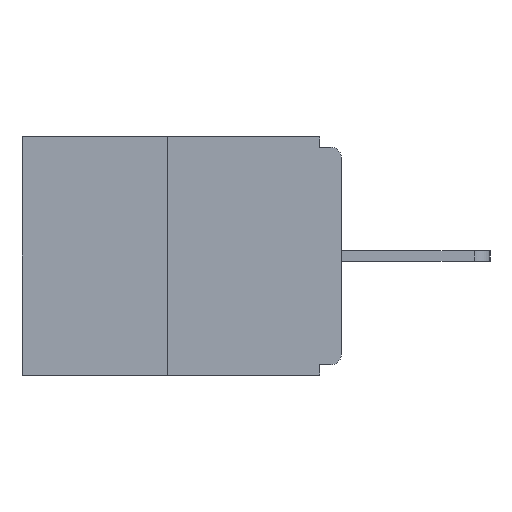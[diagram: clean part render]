
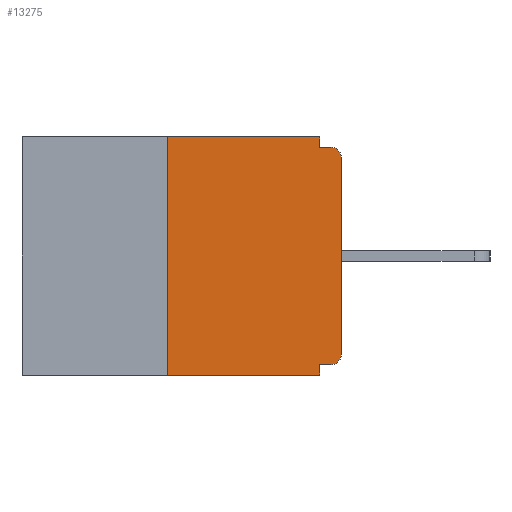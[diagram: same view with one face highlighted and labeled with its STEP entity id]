
A CAD part, left-side view. The second image highlights one B-rep face of the part: STEP entity #13275.
In plain terms, the highlighted planar face has unit normal (-1, 0, 0).
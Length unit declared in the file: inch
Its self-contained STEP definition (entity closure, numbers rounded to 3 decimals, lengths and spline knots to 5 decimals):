
#540 = EDGE_CURVE ( 'NONE', #11752, #8570, #4174, .T. ) ;
#637 = VERTEX_POINT ( 'NONE', #13024 ) ;
#772 = EDGE_CURVE ( 'NONE', #8570, #1703, #9868, .T. ) ;
#877 = DIRECTION ( 'NONE',  ( 0., 1., 0. ) ) ;
#989 = CARTESIAN_POINT ( 'NONE',  ( 0., 0.25, 0. ) ) ;
#1054 = CARTESIAN_POINT ( 'NONE',  ( 0., 0.031, -0.015 ) ) ;
#1108 = VECTOR ( 'NONE', #2287, 39.37008 ) ;
#1123 = VECTOR ( 'NONE', #13699, 39.37008 ) ;
#1276 = ORIENTED_EDGE ( 'NONE', *, *, #540, .T. ) ;
#1703 = VERTEX_POINT ( 'NONE', #7140 ) ;
#2173 = DIRECTION ( 'NONE',  ( 0., 0., 1. ) ) ;
#2223 = LINE ( 'NONE', #4532, #3395 ) ;
#2263 = ORIENTED_EDGE ( 'NONE', *, *, #12727, .F. ) ;
#2287 = DIRECTION ( 'NONE',  ( 0., 0., 1. ) ) ;
#2730 = CARTESIAN_POINT ( 'NONE',  ( 0., 0., -0.015 ) ) ;
#2786 = DIRECTION ( 'NONE',  ( 0., 0., -1. ) ) ;
#3395 = VECTOR ( 'NONE', #3484, 39.37008 ) ;
#3484 = DIRECTION ( 'NONE',  ( 0., -1., 0. ) ) ;
#3676 = VECTOR ( 'NONE', #2786, 39.37008 ) ;
#3849 = LINE ( 'NONE', #4564, #3676 ) ;
#4055 = EDGE_CURVE ( 'NONE', #8867, #12696, #3849, .T. ) ;
#4174 = LINE ( 'NONE', #11900, #1108 ) ;
#4181 = DIRECTION ( 'NONE',  ( 0., 0., -1. ) ) ;
#4206 = LINE ( 'NONE', #11777, #10544 ) ;
#4283 = CARTESIAN_POINT ( 'NONE',  ( 0., 0.031, -0.343 ) ) ;
#4357 = ORIENTED_EDGE ( 'NONE', *, *, #9547, .T. ) ;
#4532 = CARTESIAN_POINT ( 'NONE',  ( 0., 0.46, 0. ) ) ;
#4564 = CARTESIAN_POINT ( 'NONE',  ( 0., 0.031, 0. ) ) ;
#4581 = VERTEX_POINT ( 'NONE', #12182 ) ;
#4731 = AXIS2_PLACEMENT_3D ( 'NONE', #12601, #5990, #6128 ) ;
#5652 = EDGE_CURVE ( 'NONE', #637, #12661, #9093, .T. ) ;
#5801 = VECTOR ( 'NONE', #10216, 39.37008 ) ;
#5990 = DIRECTION ( 'NONE',  ( 1., 0., 0. ) ) ;
#6126 = ORIENTED_EDGE ( 'NONE', *, *, #13044, .F. ) ;
#6128 = DIRECTION ( 'NONE',  ( 0., 0., -1. ) ) ;
#6489 = LINE ( 'NONE', #10553, #7552 ) ;
#6581 = VERTEX_POINT ( 'NONE', #989 ) ;
#6760 = CARTESIAN_POINT ( 'NONE',  ( 0., 0., -0.313 ) ) ;
#6890 = ORIENTED_EDGE ( 'NONE', *, *, #9057, .F. ) ;
#7048 = CARTESIAN_POINT ( 'NONE',  ( 0., 0.015, -0.03 ) ) ;
#7140 = CARTESIAN_POINT ( 'NONE',  ( 0., 0.015, -0.015 ) ) ;
#7299 = EDGE_CURVE ( 'NONE', #4581, #637, #6489, .T. ) ;
#7317 = ORIENTED_EDGE ( 'NONE', *, *, #5652, .F. ) ;
#7338 = DIRECTION ( 'NONE',  ( -1., 0., 0. ) ) ;
#7552 = VECTOR ( 'NONE', #877, 39.37008 ) ;
#8506 = ORIENTED_EDGE ( 'NONE', *, *, #772, .T. ) ;
#8570 = VERTEX_POINT ( 'NONE', #12319 ) ;
#8647 = VECTOR ( 'NONE', #4181, 39.37008 ) ;
#8867 = VERTEX_POINT ( 'NONE', #13182 ) ;
#9057 = EDGE_CURVE ( 'NONE', #12696, #1703, #10358, .T. ) ;
#9064 = EDGE_LOOP ( 'NONE', ( #6126, #2263, #11003, #7317, #11945, #4357, #1276, #8506, #6890, #11410 ) ) ;
#9068 = DIRECTION ( 'NONE',  ( -1., 0., 0. ) ) ;
#9093 = LINE ( 'NONE', #13385, #8647 ) ;
#9357 = FACE_OUTER_BOUND ( 'NONE', #9064, .T. ) ;
#9547 = EDGE_CURVE ( 'NONE', #4581, #11752, #12759, .T. ) ;
#9552 = CARTESIAN_POINT ( 'NONE',  ( 0., 0.46, -0.343 ) ) ;
#9638 = VERTEX_POINT ( 'NONE', #12101 ) ;
#9868 = CIRCLE ( 'NONE', #11889, 0.015 ) ;
#9977 = EDGE_CURVE ( 'NONE', #9638, #12661, #10462, .T. ) ;
#10186 = DIRECTION ( 'NONE',  ( 0., 0., -1. ) ) ;
#10216 = DIRECTION ( 'NONE',  ( 0., -1., 0. ) ) ;
#10358 = LINE ( 'NONE', #2730, #5801 ) ;
#10462 = LINE ( 'NONE', #9552, #1123 ) ;
#10544 = VECTOR ( 'NONE', #2173, 39.37008 ) ;
#10553 = CARTESIAN_POINT ( 'NONE',  ( 0., 0., -0.328 ) ) ;
#11003 = ORIENTED_EDGE ( 'NONE', *, *, #9977, .T. ) ;
#11410 = ORIENTED_EDGE ( 'NONE', *, *, #4055, .F. ) ;
#11752 = VERTEX_POINT ( 'NONE', #6760 ) ;
#11777 = CARTESIAN_POINT ( 'NONE',  ( 0., 0.25, 0. ) ) ;
#11889 = AXIS2_PLACEMENT_3D ( 'NONE', #7048, #9068, #10186 ) ;
#11900 = CARTESIAN_POINT ( 'NONE',  ( 0., 0., 0. ) ) ;
#11945 = ORIENTED_EDGE ( 'NONE', *, *, #7299, .F. ) ;
#12101 = CARTESIAN_POINT ( 'NONE',  ( 0., 0.25, -0.343 ) ) ;
#12182 = CARTESIAN_POINT ( 'NONE',  ( 0., 0.015, -0.328 ) ) ;
#12319 = CARTESIAN_POINT ( 'NONE',  ( 0., 0., -0.03 ) ) ;
#12601 = CARTESIAN_POINT ( 'NONE',  ( 0., 0.46, 0. ) ) ;
#12661 = VERTEX_POINT ( 'NONE', #4283 ) ;
#12664 = CARTESIAN_POINT ( 'NONE',  ( 0., 0.015, -0.313 ) ) ;
#12696 = VERTEX_POINT ( 'NONE', #1054 ) ;
#12727 = EDGE_CURVE ( 'NONE', #9638, #6581, #4206, .T. ) ;
#12759 = CIRCLE ( 'NONE', #13203, 0.015 ) ;
#13024 = CARTESIAN_POINT ( 'NONE',  ( 0., 0.031, -0.328 ) ) ;
#13044 = EDGE_CURVE ( 'NONE', #6581, #8867, #2223, .T. ) ;
#13182 = CARTESIAN_POINT ( 'NONE',  ( 0., 0.031, 0. ) ) ;
#13203 = AXIS2_PLACEMENT_3D ( 'NONE', #12664, #7338, #13858 ) ;
#13275 = ADVANCED_FACE ( 'NONE', ( #9357 ), #13714, .F. ) ;
#13385 = CARTESIAN_POINT ( 'NONE',  ( 0., 0.031, -0.343 ) ) ;
#13699 = DIRECTION ( 'NONE',  ( 0., -1., 0. ) ) ;
#13714 = PLANE ( 'NONE',  #4731 ) ;
#13858 = DIRECTION ( 'NONE',  ( 0., 0., -1. ) ) ;
